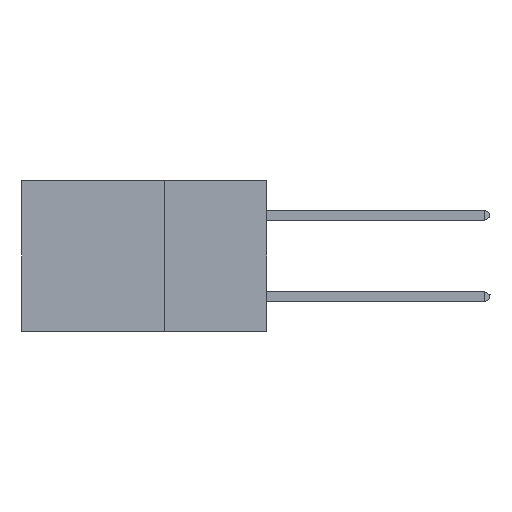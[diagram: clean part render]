
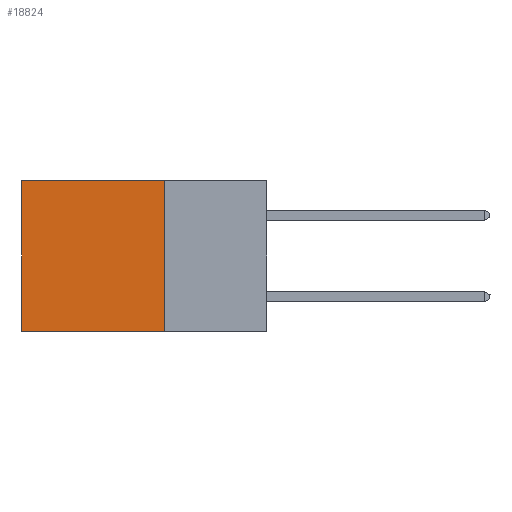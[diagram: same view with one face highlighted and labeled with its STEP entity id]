
A CAD part, left-side view. The second image highlights one B-rep face of the part: STEP entity #18824.
In plain terms, the highlighted planar face has unit normal (-1, 0, 0).
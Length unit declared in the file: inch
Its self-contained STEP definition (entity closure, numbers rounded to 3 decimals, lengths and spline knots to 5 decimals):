
#1552 = VECTOR ( 'NONE', #9372, 39.37008 ) ;
#3532 = ORIENTED_EDGE ( 'NONE', *, *, #17287, .F. ) ;
#4703 = VERTEX_POINT ( 'NONE', #36713 ) ;
#6770 = LINE ( 'NONE', #19073, #21340 ) ;
#7733 = VECTOR ( 'NONE', #10124, 39.37008 ) ;
#8013 = ORIENTED_EDGE ( 'NONE', *, *, #8059, .T. ) ;
#8059 = EDGE_CURVE ( 'NONE', #26838, #22184, #16190, .T. ) ;
#9372 = DIRECTION ( 'NONE',  ( 0., 0., -1. ) ) ;
#9905 = VECTOR ( 'NONE', #25420, 39.37008 ) ;
#10124 = DIRECTION ( 'NONE',  ( 0., 1., 0. ) ) ;
#11723 = AXIS2_PLACEMENT_3D ( 'NONE', #28793, #34644, #22927 ) ;
#12168 = CARTESIAN_POINT ( 'NONE',  ( 0.2875, 0.25, -0.37 ) ) ;
#12483 = EDGE_CURVE ( 'NONE', #22184, #4703, #19125, .T. ) ;
#13615 = FACE_OUTER_BOUND ( 'NONE', #25286, .T. ) ;
#14132 = EDGE_CURVE ( 'NONE', #26838, #15869, #27590, .T. ) ;
#15645 = DIRECTION ( 'NONE',  ( 0., 1., 0. ) ) ;
#15869 = VERTEX_POINT ( 'NONE', #12168 ) ;
#16040 = ORIENTED_EDGE ( 'NONE', *, *, #14132, .F. ) ;
#16190 = LINE ( 'NONE', #31986, #7733 ) ;
#16440 = PLANE ( 'NONE',  #11723 ) ;
#16582 = CARTESIAN_POINT ( 'NONE',  ( 0.2875, 0.6, 0. ) ) ;
#17287 = EDGE_CURVE ( 'NONE', #15869, #4703, #6770, .T. ) ;
#18824 = ADVANCED_FACE ( 'NONE', ( #13615 ), #16440, .F. ) ;
#19073 = CARTESIAN_POINT ( 'NONE',  ( 0.2875, 0.25, -0.37 ) ) ;
#19125 = LINE ( 'NONE', #26582, #9905 ) ;
#21340 = VECTOR ( 'NONE', #15645, 39.37008 ) ;
#22184 = VERTEX_POINT ( 'NONE', #16582 ) ;
#22649 = ORIENTED_EDGE ( 'NONE', *, *, #12483, .T. ) ;
#22927 = DIRECTION ( 'NONE',  ( 0., 0., -1. ) ) ;
#25286 = EDGE_LOOP ( 'NONE', ( #22649, #3532, #16040, #8013 ) ) ;
#25420 = DIRECTION ( 'NONE',  ( 0., 0., -1. ) ) ;
#26582 = CARTESIAN_POINT ( 'NONE',  ( 0.2875, 0.6, 0. ) ) ;
#26838 = VERTEX_POINT ( 'NONE', #36526 ) ;
#27590 = LINE ( 'NONE', #37061, #1552 ) ;
#28793 = CARTESIAN_POINT ( 'NONE',  ( 0.2875, 0.25, 0. ) ) ;
#31986 = CARTESIAN_POINT ( 'NONE',  ( 0.2875, 0.25, 0. ) ) ;
#34644 = DIRECTION ( 'NONE',  ( 1., 0., 0. ) ) ;
#36526 = CARTESIAN_POINT ( 'NONE',  ( 0.2875, 0.25, 0. ) ) ;
#36713 = CARTESIAN_POINT ( 'NONE',  ( 0.2875, 0.6, -0.37 ) ) ;
#37061 = CARTESIAN_POINT ( 'NONE',  ( 0.2875, 0.25, 0. ) ) ;
